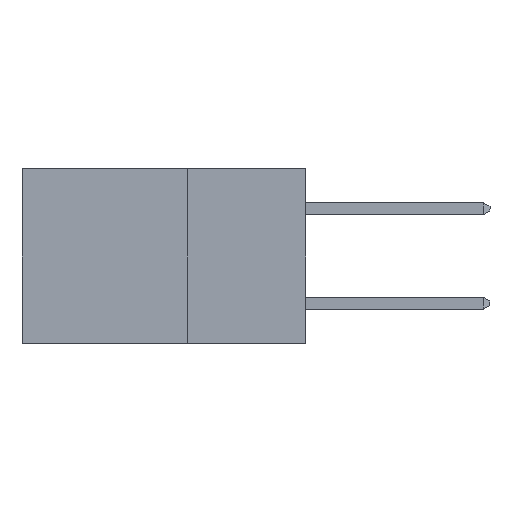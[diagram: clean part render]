
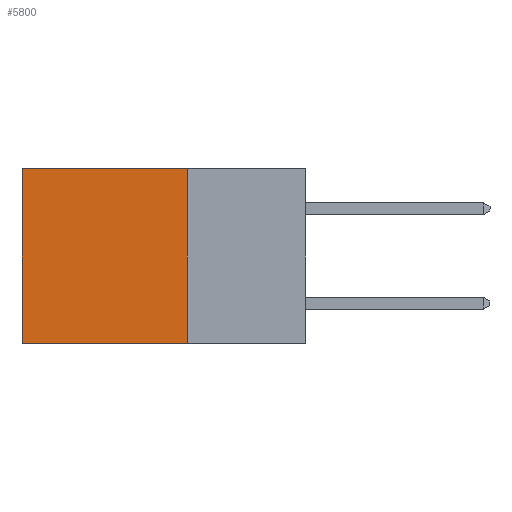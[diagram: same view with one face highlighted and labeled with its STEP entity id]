
A CAD part, left-side view. The second image highlights one B-rep face of the part: STEP entity #5800.
In plain terms, the highlighted planar face has unit normal (-1, 0, 0).
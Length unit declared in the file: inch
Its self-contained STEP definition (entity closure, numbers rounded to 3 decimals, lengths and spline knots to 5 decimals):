
#46 = LINE ( 'NONE', #9430, #742 ) ;
#78 = VECTOR ( 'NONE', #7990, 39.37008 ) ;
#193 = LINE ( 'NONE', #2488, #8243 ) ;
#248 = VERTEX_POINT ( 'NONE', #374 ) ;
#280 = CARTESIAN_POINT ( 'NONE',  ( 0.2615, 0.25, -0.37 ) ) ;
#374 = CARTESIAN_POINT ( 'NONE',  ( 0.2615, 0.25, 0. ) ) ;
#742 = VECTOR ( 'NONE', #5543, 39.37008 ) ;
#962 = FACE_OUTER_BOUND ( 'NONE', #4363, .T. ) ;
#1084 = AXIS2_PLACEMENT_3D ( 'NONE', #2336, #4095, #9315 ) ;
#1225 = DIRECTION ( 'NONE',  ( 0., 0., -1. ) ) ;
#1387 = EDGE_CURVE ( 'NONE', #4282, #4874, #193, .T. ) ;
#2203 = VECTOR ( 'NONE', #1225, 39.37008 ) ;
#2336 = CARTESIAN_POINT ( 'NONE',  ( 0.2615, 0.25, -0.37 ) ) ;
#2488 = CARTESIAN_POINT ( 'NONE',  ( 0.2615, 0.25, -0.37 ) ) ;
#2732 = CARTESIAN_POINT ( 'NONE',  ( 0.2615, 0.6, 0. ) ) ;
#3283 = DIRECTION ( 'NONE',  ( 0., 1., 0. ) ) ;
#3756 = EDGE_CURVE ( 'NONE', #248, #4282, #5810, .T. ) ;
#4095 = DIRECTION ( 'NONE',  ( 1., 0., 0. ) ) ;
#4282 = VERTEX_POINT ( 'NONE', #8451 ) ;
#4363 = EDGE_LOOP ( 'NONE', ( #6441, #4641, #6916, #9780 ) ) ;
#4641 = ORIENTED_EDGE ( 'NONE', *, *, #1387, .F. ) ;
#4874 = VERTEX_POINT ( 'NONE', #9557 ) ;
#5543 = DIRECTION ( 'NONE',  ( 0., 1., 0. ) ) ;
#5658 = CARTESIAN_POINT ( 'NONE',  ( 0.2615, 0.6, -0.37 ) ) ;
#5800 = ADVANCED_FACE ( 'NONE', ( #962 ), #6292, .F. ) ;
#5810 = LINE ( 'NONE', #280, #2203 ) ;
#6191 = EDGE_CURVE ( 'NONE', #248, #9383, #46, .T. ) ;
#6292 = PLANE ( 'NONE',  #1084 ) ;
#6441 = ORIENTED_EDGE ( 'NONE', *, *, #7737, .T. ) ;
#6916 = ORIENTED_EDGE ( 'NONE', *, *, #3756, .F. ) ;
#7737 = EDGE_CURVE ( 'NONE', #9383, #4874, #8046, .T. ) ;
#7990 = DIRECTION ( 'NONE',  ( 0., 0., -1. ) ) ;
#8046 = LINE ( 'NONE', #5658, #78 ) ;
#8243 = VECTOR ( 'NONE', #3283, 39.37008 ) ;
#8451 = CARTESIAN_POINT ( 'NONE',  ( 0.2615, 0.25, -0.37 ) ) ;
#9315 = DIRECTION ( 'NONE',  ( 0., 0., -1. ) ) ;
#9383 = VERTEX_POINT ( 'NONE', #2732 ) ;
#9430 = CARTESIAN_POINT ( 'NONE',  ( 0.2615, 0.25, 0. ) ) ;
#9557 = CARTESIAN_POINT ( 'NONE',  ( 0.2615, 0.6, -0.37 ) ) ;
#9780 = ORIENTED_EDGE ( 'NONE', *, *, #6191, .T. ) ;
